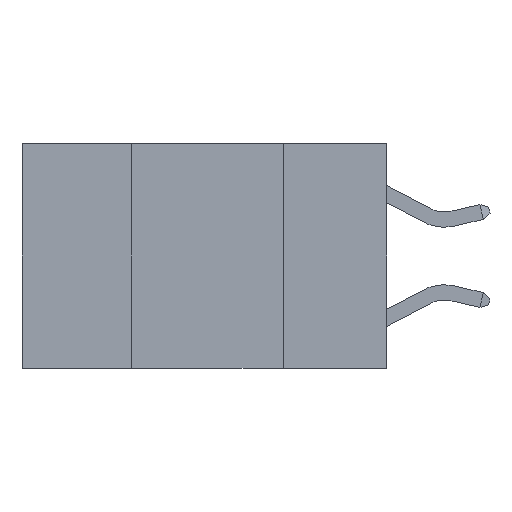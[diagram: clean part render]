
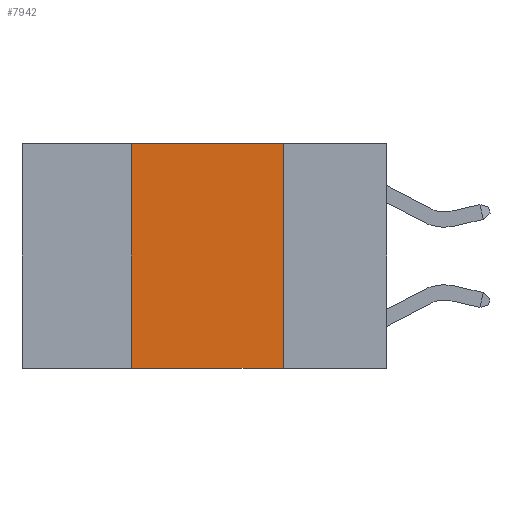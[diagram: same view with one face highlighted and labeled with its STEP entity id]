
A CAD part, left-side view. The second image highlights one B-rep face of the part: STEP entity #7942.
In plain terms, the highlighted planar face has unit normal (-1, 0, 0).
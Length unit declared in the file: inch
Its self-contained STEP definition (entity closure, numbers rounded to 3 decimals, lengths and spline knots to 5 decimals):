
#357 = CARTESIAN_POINT ( 'NONE',  ( 0., 0.17, 0. ) ) ;
#606 = CARTESIAN_POINT ( 'NONE',  ( 0., 0.42, 0. ) ) ;
#651 = CARTESIAN_POINT ( 'NONE',  ( 0., 0.17, -0.37 ) ) ;
#752 = ORIENTED_EDGE ( 'NONE', *, *, #1158, .T. ) ;
#1007 = DIRECTION ( 'NONE',  ( 0., 0., -1. ) ) ;
#1138 = LINE ( 'NONE', #2388, #11310 ) ;
#1158 = EDGE_CURVE ( 'NONE', #7025, #5652, #11125, .T. ) ;
#1923 = LINE ( 'NONE', #5982, #9271 ) ;
#2198 = CARTESIAN_POINT ( 'NONE',  ( 0., 0.6, 0. ) ) ;
#2388 = CARTESIAN_POINT ( 'NONE',  ( 0., 0.42, 0. ) ) ;
#3170 = DIRECTION ( 'NONE',  ( 0., 0., -1. ) ) ;
#3828 = EDGE_LOOP ( 'NONE', ( #7515, #7809, #10614, #752 ) ) ;
#4008 = VERTEX_POINT ( 'NONE', #357 ) ;
#4084 = PLANE ( 'NONE',  #6279 ) ;
#4566 = EDGE_CURVE ( 'NONE', #9902, #4008, #1923, .T. ) ;
#5019 = DIRECTION ( 'NONE',  ( 0., -1., 0. ) ) ;
#5652 = VERTEX_POINT ( 'NONE', #651 ) ;
#5982 = CARTESIAN_POINT ( 'NONE',  ( 0., 0.6, 0. ) ) ;
#6279 = AXIS2_PLACEMENT_3D ( 'NONE', #2198, #8912, #3170 ) ;
#6877 = EDGE_CURVE ( 'NONE', #7025, #9902, #1138, .T. ) ;
#7025 = VERTEX_POINT ( 'NONE', #11158 ) ;
#7127 = DIRECTION ( 'NONE',  ( 0., -1., 0. ) ) ;
#7515 = ORIENTED_EDGE ( 'NONE', *, *, #11267, .F. ) ;
#7724 = CARTESIAN_POINT ( 'NONE',  ( 0., 0.17, 0. ) ) ;
#7775 = LINE ( 'NONE', #7724, #9996 ) ;
#7809 = ORIENTED_EDGE ( 'NONE', *, *, #4566, .F. ) ;
#7942 = ADVANCED_FACE ( 'NONE', ( #9213 ), #4084, .F. ) ;
#8912 = DIRECTION ( 'NONE',  ( 1., 0., 0. ) ) ;
#9037 = CARTESIAN_POINT ( 'NONE',  ( 0., 0.6, -0.37 ) ) ;
#9098 = DIRECTION ( 'NONE',  ( 0., 0., 1. ) ) ;
#9213 = FACE_OUTER_BOUND ( 'NONE', #3828, .T. ) ;
#9271 = VECTOR ( 'NONE', #5019, 39.37008 ) ;
#9902 = VERTEX_POINT ( 'NONE', #606 ) ;
#9996 = VECTOR ( 'NONE', #1007, 39.37008 ) ;
#10614 = ORIENTED_EDGE ( 'NONE', *, *, #6877, .F. ) ;
#10818 = VECTOR ( 'NONE', #7127, 39.37008 ) ;
#11125 = LINE ( 'NONE', #9037, #10818 ) ;
#11158 = CARTESIAN_POINT ( 'NONE',  ( 0., 0.42, -0.37 ) ) ;
#11267 = EDGE_CURVE ( 'NONE', #4008, #5652, #7775, .T. ) ;
#11310 = VECTOR ( 'NONE', #9098, 39.37008 ) ;
